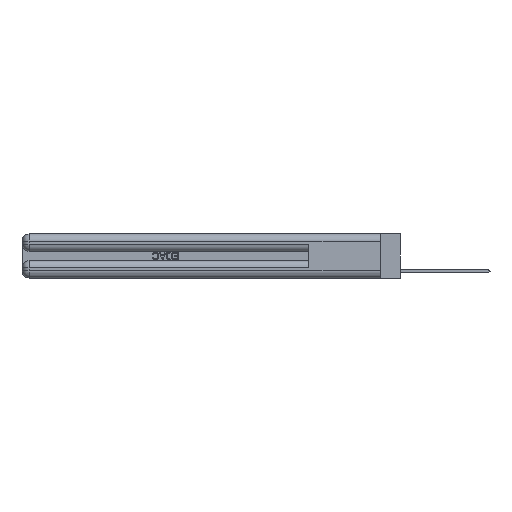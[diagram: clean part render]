
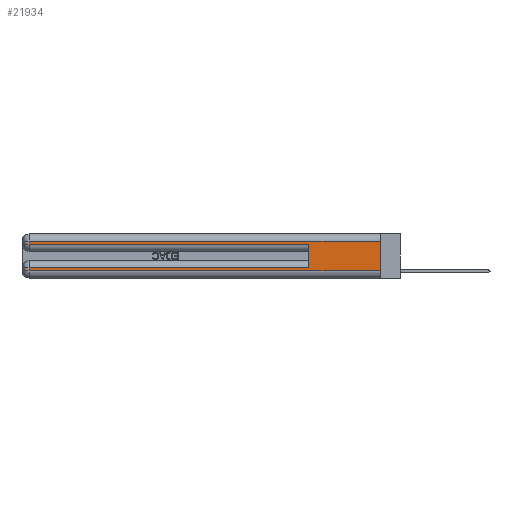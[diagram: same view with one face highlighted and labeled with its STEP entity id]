
A CAD part, left-side view. The second image highlights one B-rep face of the part: STEP entity #21934.
In plain terms, the highlighted planar face has unit normal (-1, 0, 0).
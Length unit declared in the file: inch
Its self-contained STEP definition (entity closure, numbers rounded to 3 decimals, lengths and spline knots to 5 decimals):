
#261 = VERTEX_POINT ( 'NONE', #10425 ) ;
#961 = VERTEX_POINT ( 'NONE', #23277 ) ;
#1211 = VECTOR ( 'NONE', #18407, 39.37008 ) ;
#1416 = LINE ( 'NONE', #28121, #26285 ) ;
#1825 = DIRECTION ( 'NONE',  ( 0., 1., 0. ) ) ;
#1925 = CARTESIAN_POINT ( 'NONE',  ( 0., 2.94, 0.31 ) ) ;
#2165 = EDGE_CURVE ( 'NONE', #261, #961, #19711, .T. ) ;
#2560 = LINE ( 'NONE', #17212, #4940 ) ;
#2637 = CARTESIAN_POINT ( 'NONE',  ( 0., 2.94, 0.285 ) ) ;
#3289 = EDGE_CURVE ( 'NONE', #15753, #961, #1416, .T. ) ;
#3381 = ORIENTED_EDGE ( 'NONE', *, *, #9145, .T. ) ;
#3546 = ORIENTED_EDGE ( 'NONE', *, *, #6686, .T. ) ;
#3683 = ORIENTED_EDGE ( 'NONE', *, *, #17221, .F. ) ;
#4413 = DIRECTION ( 'NONE',  ( 0., 0., 1. ) ) ;
#4905 = FACE_OUTER_BOUND ( 'NONE', #14899, .T. ) ;
#4940 = VECTOR ( 'NONE', #12370, 39.37008 ) ;
#5127 = VECTOR ( 'NONE', #4413, 39.37008 ) ;
#5679 = CARTESIAN_POINT ( 'NONE',  ( 0., 0.6, 0.085 ) ) ;
#5842 = VERTEX_POINT ( 'NONE', #5679 ) ;
#6686 = EDGE_CURVE ( 'NONE', #7792, #6775, #30819, .T. ) ;
#6775 = VERTEX_POINT ( 'NONE', #2637 ) ;
#7607 = DIRECTION ( 'NONE',  ( 0., -1., 0. ) ) ;
#7792 = VERTEX_POINT ( 'NONE', #1925 ) ;
#9145 = EDGE_CURVE ( 'NONE', #6775, #17651, #2560, .T. ) ;
#9874 = EDGE_CURVE ( 'NONE', #5842, #29489, #11292, .T. ) ;
#10425 = CARTESIAN_POINT ( 'NONE',  ( 0., 2.94, 0.06 ) ) ;
#11026 = VECTOR ( 'NONE', #18917, 39.37008 ) ;
#11111 = ORIENTED_EDGE ( 'NONE', *, *, #18645, .T. ) ;
#11292 = LINE ( 'NONE', #21138, #30741 ) ;
#11345 = ORIENTED_EDGE ( 'NONE', *, *, #9874, .T. ) ;
#11986 = PLANE ( 'NONE',  #12149 ) ;
#12149 = AXIS2_PLACEMENT_3D ( 'NONE', #14578, #21978, #28911 ) ;
#12270 = CARTESIAN_POINT ( 'NONE',  ( 0., 0., 0.31 ) ) ;
#12370 = DIRECTION ( 'NONE',  ( 0., -1., 0. ) ) ;
#13409 = CARTESIAN_POINT ( 'NONE',  ( 0., 0., 0.31 ) ) ;
#13497 = ORIENTED_EDGE ( 'NONE', *, *, #31580, .T. ) ;
#14578 = CARTESIAN_POINT ( 'NONE',  ( 0., 0., 0.37 ) ) ;
#14899 = EDGE_LOOP ( 'NONE', ( #22077, #11111, #3546, #3381, #3683, #11345, #13497, #15849 ) ) ;
#15753 = VERTEX_POINT ( 'NONE', #12270 ) ;
#15849 = ORIENTED_EDGE ( 'NONE', *, *, #2165, .T. ) ;
#17212 = CARTESIAN_POINT ( 'NONE',  ( 0., 0., 0.285 ) ) ;
#17221 = EDGE_CURVE ( 'NONE', #5842, #17651, #29376, .T. ) ;
#17651 = VERTEX_POINT ( 'NONE', #21443 ) ;
#18407 = DIRECTION ( 'NONE',  ( 0., 1., 0. ) ) ;
#18645 = EDGE_CURVE ( 'NONE', #15753, #7792, #26282, .T. ) ;
#18687 = LINE ( 'NONE', #21251, #25590 ) ;
#18917 = DIRECTION ( 'NONE',  ( 0., 0., -1. ) ) ;
#19711 = LINE ( 'NONE', #21653, #20130 ) ;
#20130 = VECTOR ( 'NONE', #7607, 39.37008 ) ;
#20578 = DIRECTION ( 'NONE',  ( 0., 0., -1. ) ) ;
#21138 = CARTESIAN_POINT ( 'NONE',  ( 0., 0., 0.085 ) ) ;
#21251 = CARTESIAN_POINT ( 'NONE',  ( 0., 2.94, 0.37 ) ) ;
#21316 = CARTESIAN_POINT ( 'NONE',  ( 0., 2.94, 0.37 ) ) ;
#21443 = CARTESIAN_POINT ( 'NONE',  ( 0., 0.6, 0.285 ) ) ;
#21652 = CARTESIAN_POINT ( 'NONE',  ( 0., 2.94, 0.085 ) ) ;
#21653 = CARTESIAN_POINT ( 'NONE',  ( 0., 0., 0.06 ) ) ;
#21934 = ADVANCED_FACE ( 'NONE', ( #4905 ), #11986, .F. ) ;
#21978 = DIRECTION ( 'NONE',  ( 1., 0., 0. ) ) ;
#22077 = ORIENTED_EDGE ( 'NONE', *, *, #3289, .F. ) ;
#23277 = CARTESIAN_POINT ( 'NONE',  ( 0., 0., 0.06 ) ) ;
#23819 = DIRECTION ( 'NONE',  ( 0., 0., -1. ) ) ;
#25590 = VECTOR ( 'NONE', #23819, 39.37008 ) ;
#26282 = LINE ( 'NONE', #13409, #1211 ) ;
#26285 = VECTOR ( 'NONE', #20578, 39.37008 ) ;
#28121 = CARTESIAN_POINT ( 'NONE',  ( 0., 0., 0.37 ) ) ;
#28911 = DIRECTION ( 'NONE',  ( 0., 0., -1. ) ) ;
#29049 = CARTESIAN_POINT ( 'NONE',  ( 0., 0.6, 0.145 ) ) ;
#29376 = LINE ( 'NONE', #29049, #5127 ) ;
#29489 = VERTEX_POINT ( 'NONE', #21652 ) ;
#30741 = VECTOR ( 'NONE', #1825, 39.37008 ) ;
#30819 = LINE ( 'NONE', #21316, #11026 ) ;
#31580 = EDGE_CURVE ( 'NONE', #29489, #261, #18687, .T. ) ;
